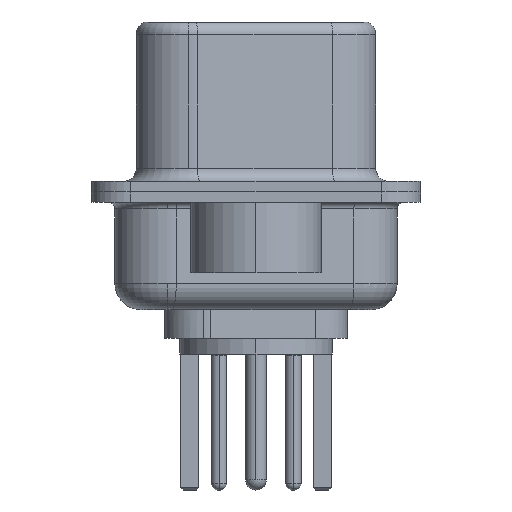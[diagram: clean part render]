
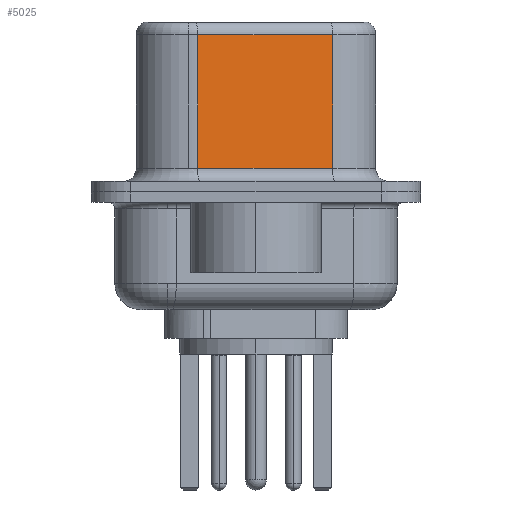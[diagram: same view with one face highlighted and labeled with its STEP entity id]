
A CAD part, left-side view. The second image highlights one B-rep face of the part: STEP entity #5025.
In plain terms, the highlighted planar face has unit normal (-0.985, -0.174, 0).
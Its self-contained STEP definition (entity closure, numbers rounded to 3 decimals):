
#264 = LINE ( 'NONE', #7853, #3753 ) ;
#297 = CARTESIAN_POINT ( 'NONE',  ( 4.565, -2.927, 6.02 ) ) ;
#937 = EDGE_CURVE ( 'NONE', #17706, #13328, #6559, .T. ) ;
#1274 = DIRECTION ( 'NONE',  ( 0.174, -0.985, 0. ) ) ;
#1288 = DIRECTION ( 'NONE',  ( 0., 0., -1. ) ) ;
#2364 = CARTESIAN_POINT ( 'NONE',  ( 3.655, 2.233, 6.02 ) ) ;
#3220 = DIRECTION ( 'NONE',  ( -0.174, 0.985, 0. ) ) ;
#3550 = CARTESIAN_POINT ( 'NONE',  ( 4.565, -2.927, 0.9 ) ) ;
#3607 = VECTOR ( 'NONE', #1288, 1000. ) ;
#3753 = VECTOR ( 'NONE', #1274, 1000. ) ;
#4019 = LINE ( 'NONE', #8425, #3607 ) ;
#4730 = DIRECTION ( 'NONE',  ( -0.174, 0.985, 0. ) ) ;
#4830 = CARTESIAN_POINT ( 'NONE',  ( 4.565, -2.927, 6.02 ) ) ;
#4872 = FACE_OUTER_BOUND ( 'NONE', #13110, .T. ) ;
#4973 = VERTEX_POINT ( 'NONE', #17925 ) ;
#5025 = ADVANCED_FACE ( 'NONE', ( #4872 ), #15052, .F. ) ;
#5713 = EDGE_CURVE ( 'NONE', #13328, #4973, #4019, .T. ) ;
#6559 = LINE ( 'NONE', #297, #13725 ) ;
#6883 = AXIS2_PLACEMENT_3D ( 'NONE', #12352, #12314, #4730 ) ;
#7853 = CARTESIAN_POINT ( 'NONE',  ( 4.565, -2.927, 0.9 ) ) ;
#8425 = CARTESIAN_POINT ( 'NONE',  ( 3.655, 2.233, 6.52 ) ) ;
#10883 = EDGE_CURVE ( 'NONE', #4973, #13889, #264, .T. ) ;
#12314 = DIRECTION ( 'NONE',  ( 0.985, 0.174, 0. ) ) ;
#12352 = CARTESIAN_POINT ( 'NONE',  ( 4.565, -2.927, 6.52 ) ) ;
#13110 = EDGE_LOOP ( 'NONE', ( #13248, #17689, #14739, #18126 ) ) ;
#13248 = ORIENTED_EDGE ( 'NONE', *, *, #13892, .F. ) ;
#13328 = VERTEX_POINT ( 'NONE', #2364 ) ;
#13725 = VECTOR ( 'NONE', #3220, 1000. ) ;
#13889 = VERTEX_POINT ( 'NONE', #3550 ) ;
#13892 = EDGE_CURVE ( 'NONE', #17706, #13889, #13928, .T. ) ;
#13928 = LINE ( 'NONE', #14766, #17462 ) ;
#14739 = ORIENTED_EDGE ( 'NONE', *, *, #5713, .T. ) ;
#14766 = CARTESIAN_POINT ( 'NONE',  ( 4.565, -2.927, 6.52 ) ) ;
#15052 = PLANE ( 'NONE',  #6883 ) ;
#16308 = DIRECTION ( 'NONE',  ( 0., 0., -1. ) ) ;
#17462 = VECTOR ( 'NONE', #16308, 1000. ) ;
#17689 = ORIENTED_EDGE ( 'NONE', *, *, #937, .T. ) ;
#17706 = VERTEX_POINT ( 'NONE', #4830 ) ;
#17925 = CARTESIAN_POINT ( 'NONE',  ( 3.655, 2.233, 0.9 ) ) ;
#18126 = ORIENTED_EDGE ( 'NONE', *, *, #10883, .T. ) ;
